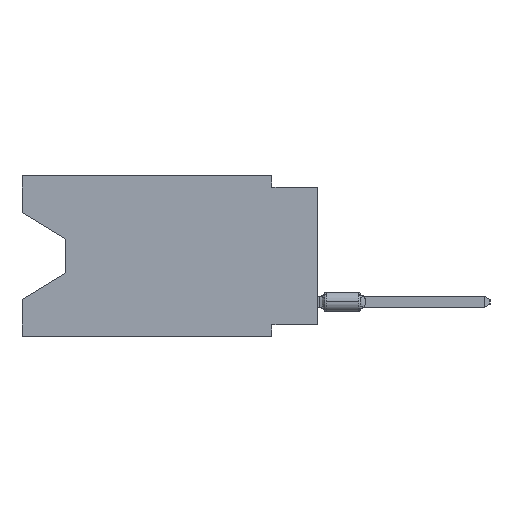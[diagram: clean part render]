
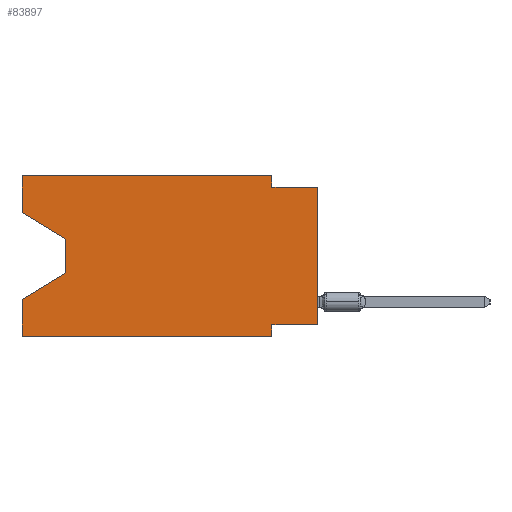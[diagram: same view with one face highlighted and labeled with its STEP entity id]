
A CAD part, left-side view. The second image highlights one B-rep face of the part: STEP entity #83897.
In plain terms, the highlighted planar face has unit normal (-1, 0, 0).
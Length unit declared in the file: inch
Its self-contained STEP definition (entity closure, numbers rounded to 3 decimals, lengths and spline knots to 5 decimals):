
#1474 = CARTESIAN_POINT ( 'NONE',  ( 0., 0.645, -0.35 ) ) ;
#4575 = CARTESIAN_POINT ( 'NONE',  ( 0., 0.1, -0.025 ) ) ;
#5591 = ORIENTED_EDGE ( 'NONE', *, *, #77002, .F. ) ;
#5928 = DIRECTION ( 'NONE',  ( 0., -1., 0. ) ) ;
#8141 = VECTOR ( 'NONE', #50925, 39.37008 ) ;
#8808 = LINE ( 'NONE', #33168, #89472 ) ;
#10712 = DIRECTION ( 'NONE',  ( 0., -1., 0. ) ) ;
#11788 = CARTESIAN_POINT ( 'NONE',  ( 0., 0.645, 0. ) ) ;
#14153 = CARTESIAN_POINT ( 'NONE',  ( 0., 0., 0. ) ) ;
#14566 = ORIENTED_EDGE ( 'NONE', *, *, #56825, .T. ) ;
#19159 = VERTEX_POINT ( 'NONE', #76290 ) ;
#21813 = VERTEX_POINT ( 'NONE', #34748 ) ;
#22296 = VERTEX_POINT ( 'NONE', #89212 ) ;
#22898 = VECTOR ( 'NONE', #28479, 39.37008 ) ;
#23962 = ORIENTED_EDGE ( 'NONE', *, *, #32161, .T. ) ;
#24839 = EDGE_CURVE ( 'NONE', #33323, #22296, #91557, .T. ) ;
#26905 = VECTOR ( 'NONE', #78449, 39.37008 ) ;
#27577 = VECTOR ( 'NONE', #46257, 39.37008 ) ;
#27828 = EDGE_LOOP ( 'NONE', ( #93523, #23962, #14566, #46045, #31645, #65222, #54073, #89036, #44173, #62866, #36134, #5591 ) ) ;
#28479 = DIRECTION ( 'NONE',  ( 0., 0., 1. ) ) ;
#29185 = VECTOR ( 'NONE', #84585, 39.37008 ) ;
#29368 = CARTESIAN_POINT ( 'NONE',  ( 0., 0.55, -0.138 ) ) ;
#31645 = ORIENTED_EDGE ( 'NONE', *, *, #102337, .T. ) ;
#32161 = EDGE_CURVE ( 'NONE', #52995, #21813, #95547, .T. ) ;
#32775 = DIRECTION ( 'NONE',  ( 0., 0., 1. ) ) ;
#32961 = EDGE_CURVE ( 'NONE', #34846, #96057, #8808, .T. ) ;
#33051 = CARTESIAN_POINT ( 'NONE',  ( 0., 0.645, -0.35 ) ) ;
#33168 = CARTESIAN_POINT ( 'NONE',  ( 0., 0.1, 0. ) ) ;
#33323 = VERTEX_POINT ( 'NONE', #36921 ) ;
#33771 = LINE ( 'NONE', #84058, #99784 ) ;
#34748 = CARTESIAN_POINT ( 'NONE',  ( 0., 0.55, -0.212 ) ) ;
#34846 = VERTEX_POINT ( 'NONE', #68445 ) ;
#36134 = ORIENTED_EDGE ( 'NONE', *, *, #95435, .F. ) ;
#36921 = CARTESIAN_POINT ( 'NONE',  ( 0., 0., -0.325 ) ) ;
#38543 = VECTOR ( 'NONE', #10712, 39.37008 ) ;
#39171 = VERTEX_POINT ( 'NONE', #47736 ) ;
#41657 = LINE ( 'NONE', #50111, #29185 ) ;
#44173 = ORIENTED_EDGE ( 'NONE', *, *, #45942, .F. ) ;
#44310 = CARTESIAN_POINT ( 'NONE',  ( 0., 0.645, 0. ) ) ;
#45942 = EDGE_CURVE ( 'NONE', #96057, #22296, #53660, .T. ) ;
#46045 = ORIENTED_EDGE ( 'NONE', *, *, #68680, .F. ) ;
#46257 = DIRECTION ( 'NONE',  ( 0., 0., 1. ) ) ;
#46629 = CARTESIAN_POINT ( 'NONE',  ( 0., 0.645, -0.08025 ) ) ;
#47736 = CARTESIAN_POINT ( 'NONE',  ( 0., 0.1, -0.325 ) ) ;
#50111 = CARTESIAN_POINT ( 'NONE',  ( 0., 0.1, -0.35 ) ) ;
#50617 = CARTESIAN_POINT ( 'NONE',  ( 0., 0.1, -0.35 ) ) ;
#50925 = DIRECTION ( 'NONE',  ( 0., 0., -1. ) ) ;
#52995 = VERTEX_POINT ( 'NONE', #29368 ) ;
#53230 = EDGE_CURVE ( 'NONE', #80660, #52995, #104196, .T. ) ;
#53660 = LINE ( 'NONE', #78540, #38543 ) ;
#54073 = ORIENTED_EDGE ( 'NONE', *, *, #84777, .F. ) ;
#55461 = DIRECTION ( 'NONE',  ( 0., 0., -1. ) ) ;
#55646 = EDGE_CURVE ( 'NONE', #39171, #99720, #41657, .T. ) ;
#56825 = EDGE_CURVE ( 'NONE', #21813, #19159, #33771, .T. ) ;
#59340 = VECTOR ( 'NONE', #32775, 39.37008 ) ;
#61279 = CARTESIAN_POINT ( 'NONE',  ( 0., 0.645, 0. ) ) ;
#62866 = ORIENTED_EDGE ( 'NONE', *, *, #32961, .F. ) ;
#62876 = DIRECTION ( 'NONE',  ( 0., -0.855, -0.519 ) ) ;
#63335 = VERTEX_POINT ( 'NONE', #1474 ) ;
#65222 = ORIENTED_EDGE ( 'NONE', *, *, #55646, .F. ) ;
#68445 = CARTESIAN_POINT ( 'NONE',  ( 0., 0.1, 0. ) ) ;
#68680 = EDGE_CURVE ( 'NONE', #63335, #19159, #95744, .T. ) ;
#70873 = DIRECTION ( 'NONE',  ( 1., 0., 0. ) ) ;
#73318 = VECTOR ( 'NONE', #97793, 39.37008 ) ;
#75020 = DIRECTION ( 'NONE',  ( 0., 0.855, -0.519 ) ) ;
#75677 = AXIS2_PLACEMENT_3D ( 'NONE', #61279, #70873, #55461 ) ;
#76290 = CARTESIAN_POINT ( 'NONE',  ( 0., 0.645, -0.26975 ) ) ;
#77002 = EDGE_CURVE ( 'NONE', #80660, #84540, #81271, .T. ) ;
#77756 = DIRECTION ( 'NONE',  ( 0., 0., -1. ) ) ;
#77806 = VECTOR ( 'NONE', #62876, 39.37008 ) ;
#77905 = LINE ( 'NONE', #111827, #26905 ) ;
#78449 = DIRECTION ( 'NONE',  ( 0., 1., 0. ) ) ;
#78540 = CARTESIAN_POINT ( 'NONE',  ( 0., 0., -0.025 ) ) ;
#80660 = VERTEX_POINT ( 'NONE', #46629 ) ;
#81271 = LINE ( 'NONE', #11788, #27577 ) ;
#82014 = PLANE ( 'NONE',  #75677 ) ;
#83897 = ADVANCED_FACE ( 'NONE', ( #96336 ), #82014, .F. ) ;
#84058 = CARTESIAN_POINT ( 'NONE',  ( 0., 0.55, -0.212 ) ) ;
#84540 = VERTEX_POINT ( 'NONE', #98333 ) ;
#84585 = DIRECTION ( 'NONE',  ( 0., 0., -1. ) ) ;
#84777 = EDGE_CURVE ( 'NONE', #33323, #39171, #77905, .T. ) ;
#87238 = CARTESIAN_POINT ( 'NONE',  ( 0., 0.645, -0.08025 ) ) ;
#89036 = ORIENTED_EDGE ( 'NONE', *, *, #24839, .T. ) ;
#89212 = CARTESIAN_POINT ( 'NONE',  ( 0., 0., -0.025 ) ) ;
#89472 = VECTOR ( 'NONE', #77756, 39.37008 ) ;
#90972 = CARTESIAN_POINT ( 'NONE',  ( 0., 0.645, 0. ) ) ;
#91279 = LINE ( 'NONE', #33051, #108122 ) ;
#91557 = LINE ( 'NONE', #14153, #59340 ) ;
#93523 = ORIENTED_EDGE ( 'NONE', *, *, #53230, .T. ) ;
#95435 = EDGE_CURVE ( 'NONE', #84540, #34846, #107376, .T. ) ;
#95547 = LINE ( 'NONE', #104593, #8141 ) ;
#95744 = LINE ( 'NONE', #44310, #22898 ) ;
#96057 = VERTEX_POINT ( 'NONE', #4575 ) ;
#96336 = FACE_OUTER_BOUND ( 'NONE', #27828, .T. ) ;
#97793 = DIRECTION ( 'NONE',  ( 0., -1., 0. ) ) ;
#98333 = CARTESIAN_POINT ( 'NONE',  ( 0., 0.645, 0. ) ) ;
#99720 = VERTEX_POINT ( 'NONE', #50617 ) ;
#99784 = VECTOR ( 'NONE', #75020, 39.37008 ) ;
#102337 = EDGE_CURVE ( 'NONE', #63335, #99720, #91279, .T. ) ;
#104196 = LINE ( 'NONE', #87238, #77806 ) ;
#104593 = CARTESIAN_POINT ( 'NONE',  ( 0., 0.55, -0.138 ) ) ;
#107376 = LINE ( 'NONE', #90972, #73318 ) ;
#108122 = VECTOR ( 'NONE', #5928, 39.37008 ) ;
#111827 = CARTESIAN_POINT ( 'NONE',  ( 0., 0., -0.325 ) ) ;
